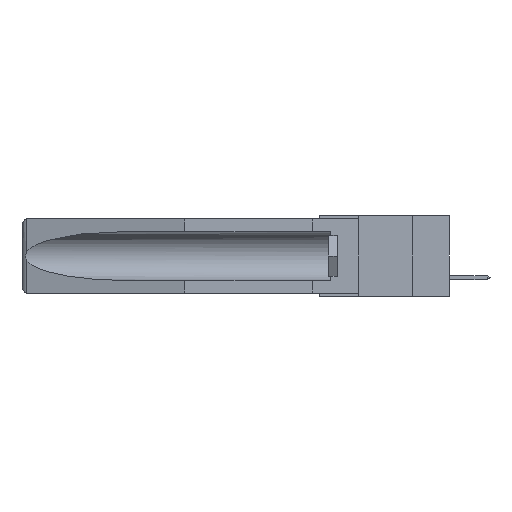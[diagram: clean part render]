
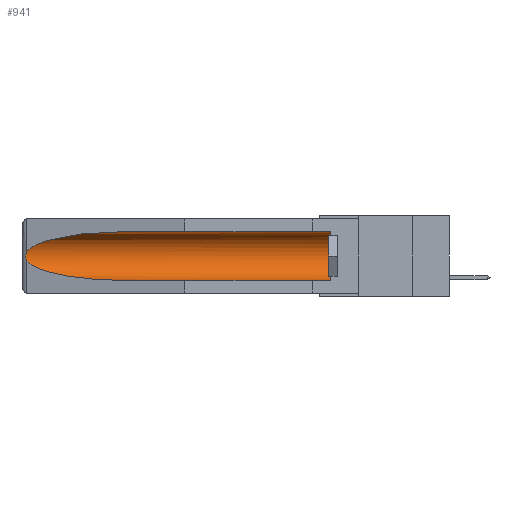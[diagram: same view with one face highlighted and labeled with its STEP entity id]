
A CAD part, left-side view. The second image highlights one B-rep face of the part: STEP entity #941.
In plain terms, the highlighted cylindrical face has radius 2.857 mm (diameter 5.715 mm), a partial arc.
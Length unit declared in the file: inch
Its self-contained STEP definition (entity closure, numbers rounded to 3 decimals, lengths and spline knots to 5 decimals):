
#77 = B_SPLINE_CURVE_WITH_KNOTS ( 'NONE', 3,
 ( #19457, #596, #2988, #13611, #13450, #6924, #26468, #26302, #15608, #22353 ),
 .UNSPECIFIED., .F., .F.,
 ( 4, 2, 2, 2, 4 ),
 ( 0., 0.00029, 0.00058, 0.00087, 0.00117 ),
 .UNSPECIFIED. ) ;
#596 = CARTESIAN_POINT ( 'NONE',  ( 0.26597, 1.52961, -0.15275 ) ) ;
#625 = ORIENTED_EDGE ( 'NONE', *, *, #26443, .T. ) ;
#941 = ADVANCED_FACE ( 'NONE', ( #17197 ), #24258, .F. ) ;
#1350 = DIRECTION ( 'NONE',  ( 0., 1., 0. ) ) ;
#2422 = CARTESIAN_POINT ( 'NONE',  ( 0.26537, 1.52718, -0.19328 ) ) ;
#2434 = CARTESIAN_POINT ( 'NONE',  ( 0.21114, 1.30732, -0.059 ) ) ;
#2988 = CARTESIAN_POINT ( 'NONE',  ( 0.26654, 1.53092, -0.15636 ) ) ;
#3375 = DIRECTION ( 'NONE',  ( 0., -1., 0. ) ) ;
#3521 = VERTEX_POINT ( 'NONE', #6267 ) ;
#4302 = LINE ( 'NONE', #12931, #8343 ) ;
#6026 = ORIENTED_EDGE ( 'NONE', *, *, #15351, .T. ) ;
#6267 = CARTESIAN_POINT ( 'NONE',  ( 0.155, 1.07973, -0.284 ) ) ;
#6924 = CARTESIAN_POINT ( 'NONE',  ( 0.2675, 1.53308, -0.17534 ) ) ;
#7536 = CARTESIAN_POINT ( 'NONE',  ( 0.26537, 1.52718, -0.14972 ) ) ;
#8190 = EDGE_LOOP ( 'NONE', ( #25866, #8594, #6026, #9564, #21188, #625 ) ) ;
#8343 = VECTOR ( 'NONE', #25718, 39.37008 ) ;
#8431 = CIRCLE ( 'NONE', #21527, 0.1125 ) ;
#8530 = EDGE_CURVE ( 'NONE', #27376, #10854, #8431, .T. ) ;
#8552 = DIRECTION ( 'NONE',  ( 0., 1., 0. ) ) ;
#8594 = ORIENTED_EDGE ( 'NONE', *, *, #18098, .T. ) ;
#8951 = CARTESIAN_POINT ( 'NONE',  ( 0.25451, 1.48313, -0.24835 ) ) ;
#9564 = ORIENTED_EDGE ( 'NONE', *, *, #11526, .F. ) ;
#9765 = CARTESIAN_POINT ( 'NONE',  ( 0.155, 0.126, -0.1715 ) ) ;
#10854 = VERTEX_POINT ( 'NONE', #26150 ) ;
#10927 = CARTESIAN_POINT ( 'NONE',  ( 0.26537, 1.52718, -0.14972 ) ) ;
#11306 = CARTESIAN_POINT ( 'NONE',  ( 0.155, 1.07973, -0.059 ) ) ;
#11526 = EDGE_CURVE ( 'NONE', #27376, #3521, #16061, .T. ) ;
#12931 = CARTESIAN_POINT ( 'NONE',  ( 0.155, -0.30754, -0.059 ) ) ;
#13097 = DIRECTION ( 'NONE',  ( 0., 0., 1. ) ) ;
#13450 = CARTESIAN_POINT ( 'NONE',  ( 0.2675, 1.53308, -0.16763 ) ) ;
#13611 = CARTESIAN_POINT ( 'NONE',  ( 0.2673, 1.5327, -0.16383 ) ) ;
#14107 = DIRECTION ( 'NONE',  ( 0., 0., 1. ) ) ;
#15351 = EDGE_CURVE ( 'NONE', #24267, #3521, #26201, .T. ) ;
#15468 = CARTESIAN_POINT ( 'NONE',  ( 0.155, 0.126, -0.284 ) ) ;
#15608 = CARTESIAN_POINT ( 'NONE',  ( 0.26597, 1.5296, -0.19026 ) ) ;
#16061 = LINE ( 'NONE', #26865, #27803 ) ;
#17197 = FACE_OUTER_BOUND ( 'NONE', #8190, .T. ) ;
#17722 = CARTESIAN_POINT ( 'NONE',  ( 0.155, 1.07973, -0.284 ) ) ;
#18098 = EDGE_CURVE ( 'NONE', #26409, #24267, #77, .T. ) ;
#18145 = AXIS2_PLACEMENT_3D ( 'NONE', #21444, #8552, #13097 ) ;
#18803 =( BOUNDED_CURVE ( )  B_SPLINE_CURVE ( 3, ( #11306, #2434, #20147, #7536 ),
 .UNSPECIFIED., .F., .F. ) 
 B_SPLINE_CURVE_WITH_KNOTS ( ( 4, 4 ),
 ( 4.71239, 6.08839 ),
 .UNSPECIFIED. ) 
 CURVE ( )  GEOMETRIC_REPRESENTATION_ITEM ( )  RATIONAL_B_SPLINE_CURVE ( ( 1., 0.848, 0.848, 1. ) ) 
 REPRESENTATION_ITEM ( '' )  );
#19457 = CARTESIAN_POINT ( 'NONE',  ( 0.26537, 1.52718, -0.14972 ) ) ;
#19602 = EDGE_CURVE ( 'NONE', #21047, #26409, #18803, .T. ) ;
#20091 = CARTESIAN_POINT ( 'NONE',  ( 0.155, 1.07973, -0.059 ) ) ;
#20147 = CARTESIAN_POINT ( 'NONE',  ( 0.25451, 1.48313, -0.09465 ) ) ;
#21047 = VERTEX_POINT ( 'NONE', #20091 ) ;
#21188 = ORIENTED_EDGE ( 'NONE', *, *, #8530, .T. ) ;
#21444 = CARTESIAN_POINT ( 'NONE',  ( 0.155, -0.30754, -0.1715 ) ) ;
#21527 = AXIS2_PLACEMENT_3D ( 'NONE', #9765, #3375, #14107 ) ;
#22353 = CARTESIAN_POINT ( 'NONE',  ( 0.26537, 1.52718, -0.19328 ) ) ;
#24019 = CARTESIAN_POINT ( 'NONE',  ( 0.21114, 1.30732, -0.284 ) ) ;
#24258 = CYLINDRICAL_SURFACE ( 'NONE', #18145, 0.1125 ) ;
#24267 = VERTEX_POINT ( 'NONE', #26756 ) ;
#25718 = DIRECTION ( 'NONE',  ( 0., 1., 0. ) ) ;
#25866 = ORIENTED_EDGE ( 'NONE', *, *, #19602, .T. ) ;
#26150 = CARTESIAN_POINT ( 'NONE',  ( 0.155, 0.126, -0.059 ) ) ;
#26201 =( BOUNDED_CURVE ( )  B_SPLINE_CURVE ( 3, ( #2422, #8951, #24019, #17722 ),
 .UNSPECIFIED., .F., .F. ) 
 B_SPLINE_CURVE_WITH_KNOTS ( ( 4, 4 ),
 ( 0.1948, 1.5708 ),
 .UNSPECIFIED. ) 
 CURVE ( )  GEOMETRIC_REPRESENTATION_ITEM ( )  RATIONAL_B_SPLINE_CURVE ( ( 1., 0.848, 0.848, 1. ) ) 
 REPRESENTATION_ITEM ( '' )  );
#26302 = CARTESIAN_POINT ( 'NONE',  ( 0.26655, 1.53094, -0.18657 ) ) ;
#26409 = VERTEX_POINT ( 'NONE', #10927 ) ;
#26443 = EDGE_CURVE ( 'NONE', #10854, #21047, #4302, .T. ) ;
#26468 = CARTESIAN_POINT ( 'NONE',  ( 0.2673, 1.53269, -0.17917 ) ) ;
#26756 = CARTESIAN_POINT ( 'NONE',  ( 0.26537, 1.52718, -0.19328 ) ) ;
#26865 = CARTESIAN_POINT ( 'NONE',  ( 0.155, -0.30754, -0.284 ) ) ;
#27376 = VERTEX_POINT ( 'NONE', #15468 ) ;
#27803 = VECTOR ( 'NONE', #1350, 39.37008 ) ;
